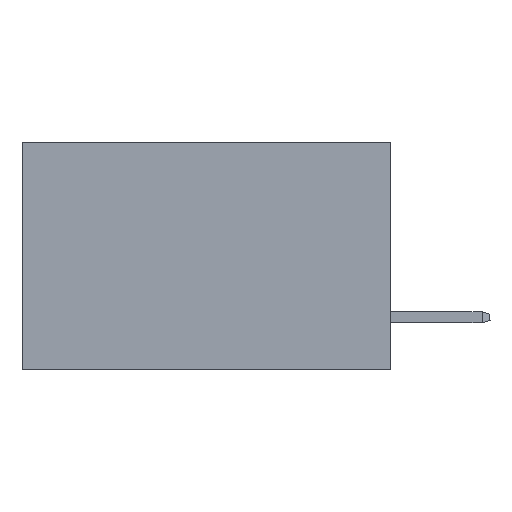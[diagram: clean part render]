
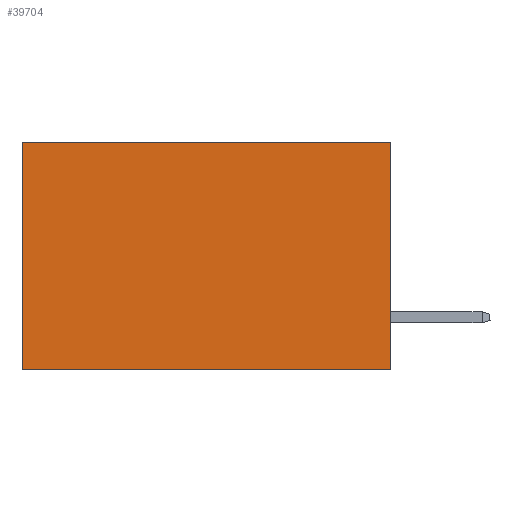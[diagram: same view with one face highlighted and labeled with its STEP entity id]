
A CAD part, left-side view. The second image highlights one B-rep face of the part: STEP entity #39704.
In plain terms, the highlighted planar face has unit normal (-1, 0, 0).
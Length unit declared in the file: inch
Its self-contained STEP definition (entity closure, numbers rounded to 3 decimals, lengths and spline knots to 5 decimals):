
#1588 = CARTESIAN_POINT ( 'NONE',  ( 0.2875, 0., 0. ) ) ;
#3426 = LINE ( 'NONE', #35936, #39644 ) ;
#4204 = PLANE ( 'NONE',  #29611 ) ;
#9386 = VECTOR ( 'NONE', #18936, 39.37008 ) ;
#10035 = DIRECTION ( 'NONE',  ( 0., 1., 0. ) ) ;
#10161 = ORIENTED_EDGE ( 'NONE', *, *, #18135, .F. ) ;
#10469 = DIRECTION ( 'NONE',  ( 0., 1., 0. ) ) ;
#11175 = VERTEX_POINT ( 'NONE', #28994 ) ;
#11546 = LINE ( 'NONE', #44077, #21572 ) ;
#17056 = VERTEX_POINT ( 'NONE', #1588 ) ;
#17361 = LINE ( 'NONE', #31386, #30822 ) ;
#18135 = EDGE_CURVE ( 'NONE', #17056, #11175, #29988, .T. ) ;
#18936 = DIRECTION ( 'NONE',  ( 0., 0., -1. ) ) ;
#19459 = VERTEX_POINT ( 'NONE', #27866 ) ;
#21340 = EDGE_CURVE ( 'NONE', #17056, #19459, #17361, .T. ) ;
#21572 = VECTOR ( 'NONE', #40154, 39.37008 ) ;
#22439 = ORIENTED_EDGE ( 'NONE', *, *, #38061, .F. ) ;
#24645 = EDGE_LOOP ( 'NONE', ( #35952, #22439, #10161, #37639 ) ) ;
#26459 = DIRECTION ( 'NONE',  ( 1., 0., 0. ) ) ;
#27361 = EDGE_CURVE ( 'NONE', #19459, #42081, #11546, .T. ) ;
#27866 = CARTESIAN_POINT ( 'NONE',  ( 0.2875, 0.6, 0. ) ) ;
#28994 = CARTESIAN_POINT ( 'NONE',  ( 0.2875, 0., -0.37 ) ) ;
#29611 = AXIS2_PLACEMENT_3D ( 'NONE', #37142, #26459, #33854 ) ;
#29988 = LINE ( 'NONE', #36571, #9386 ) ;
#30822 = VECTOR ( 'NONE', #10035, 39.37008 ) ;
#31386 = CARTESIAN_POINT ( 'NONE',  ( 0.2875, 0., 0. ) ) ;
#33854 = DIRECTION ( 'NONE',  ( 0., 0., -1. ) ) ;
#35936 = CARTESIAN_POINT ( 'NONE',  ( 0.2875, 0., -0.37 ) ) ;
#35952 = ORIENTED_EDGE ( 'NONE', *, *, #27361, .T. ) ;
#36571 = CARTESIAN_POINT ( 'NONE',  ( 0.2875, 0., 0. ) ) ;
#37142 = CARTESIAN_POINT ( 'NONE',  ( 0.2875, 0., 0. ) ) ;
#37639 = ORIENTED_EDGE ( 'NONE', *, *, #21340, .T. ) ;
#38061 = EDGE_CURVE ( 'NONE', #11175, #42081, #3426, .T. ) ;
#39644 = VECTOR ( 'NONE', #10469, 39.37008 ) ;
#39704 = ADVANCED_FACE ( 'NONE', ( #40891 ), #4204, .F. ) ;
#40154 = DIRECTION ( 'NONE',  ( 0., 0., -1. ) ) ;
#40891 = FACE_OUTER_BOUND ( 'NONE', #24645, .T. ) ;
#42081 = VERTEX_POINT ( 'NONE', #42197 ) ;
#42197 = CARTESIAN_POINT ( 'NONE',  ( 0.2875, 0.6, -0.37 ) ) ;
#44077 = CARTESIAN_POINT ( 'NONE',  ( 0.2875, 0.6, 0. ) ) ;
